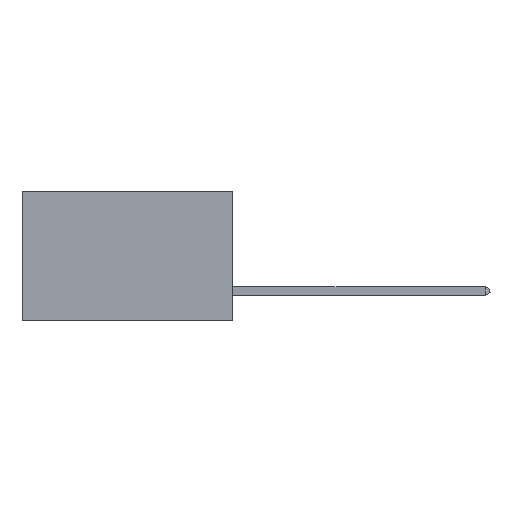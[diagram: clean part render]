
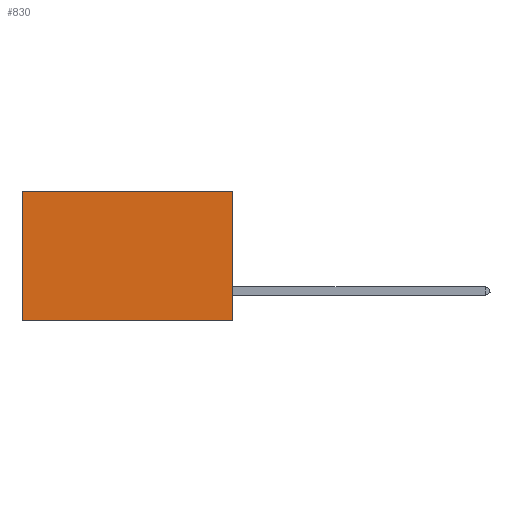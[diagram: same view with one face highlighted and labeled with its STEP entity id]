
A CAD part, left-side view. The second image highlights one B-rep face of the part: STEP entity #830.
In plain terms, the highlighted planar face has unit normal (-1, 0, 0).
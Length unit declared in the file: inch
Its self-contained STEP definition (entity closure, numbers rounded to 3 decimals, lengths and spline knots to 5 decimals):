
#830 = ADVANCED_FACE ( 'NONE', ( #8423 ), #7427, .F. ) ;
#2379 = VERTEX_POINT ( 'NONE', #4380 ) ;
#2841 = CARTESIAN_POINT ( 'NONE',  ( 0.2875, 0.6, 0. ) ) ;
#3124 = DIRECTION ( 'NONE',  ( 0., 1., 0. ) ) ;
#3214 = LINE ( 'NONE', #2841, #3964 ) ;
#3760 = EDGE_CURVE ( 'NONE', #12371, #2379, #3214, .T. ) ;
#3964 = VECTOR ( 'NONE', #4681, 39.37008 ) ;
#4380 = CARTESIAN_POINT ( 'NONE',  ( 0.2875, 0.6, -0.37 ) ) ;
#4681 = DIRECTION ( 'NONE',  ( 0., 0., -1. ) ) ;
#4777 = VERTEX_POINT ( 'NONE', #9364 ) ;
#4793 = EDGE_LOOP ( 'NONE', ( #9267, #10364, #8176, #6289 ) ) ;
#5035 = CARTESIAN_POINT ( 'NONE',  ( 0.2875, 0., -0.37 ) ) ;
#5230 = VECTOR ( 'NONE', #6561, 39.37008 ) ;
#5397 = CARTESIAN_POINT ( 'NONE',  ( 0.2875, 0., 0. ) ) ;
#5684 = VECTOR ( 'NONE', #11351, 39.37008 ) ;
#5814 = EDGE_CURVE ( 'NONE', #4777, #7488, #6009, .T. ) ;
#6009 = LINE ( 'NONE', #5397, #5684 ) ;
#6289 = ORIENTED_EDGE ( 'NONE', *, *, #12443, .T. ) ;
#6561 = DIRECTION ( 'NONE',  ( 0., 1., 0. ) ) ;
#6941 = AXIS2_PLACEMENT_3D ( 'NONE', #10407, #7470, #9533 ) ;
#7427 = PLANE ( 'NONE',  #6941 ) ;
#7435 = CARTESIAN_POINT ( 'NONE',  ( 0.2875, 0.6, 0. ) ) ;
#7470 = DIRECTION ( 'NONE',  ( 1., 0., 0. ) ) ;
#7488 = VERTEX_POINT ( 'NONE', #5035 ) ;
#8176 = ORIENTED_EDGE ( 'NONE', *, *, #5814, .F. ) ;
#8423 = FACE_OUTER_BOUND ( 'NONE', #4793, .T. ) ;
#8482 = CARTESIAN_POINT ( 'NONE',  ( 0.2875, 0., 0. ) ) ;
#9236 = EDGE_CURVE ( 'NONE', #7488, #2379, #10485, .T. ) ;
#9267 = ORIENTED_EDGE ( 'NONE', *, *, #3760, .T. ) ;
#9364 = CARTESIAN_POINT ( 'NONE',  ( 0.2875, 0., 0. ) ) ;
#9533 = DIRECTION ( 'NONE',  ( 0., 0., -1. ) ) ;
#10364 = ORIENTED_EDGE ( 'NONE', *, *, #9236, .F. ) ;
#10407 = CARTESIAN_POINT ( 'NONE',  ( 0.2875, 0., 0. ) ) ;
#10485 = LINE ( 'NONE', #10801, #11086 ) ;
#10801 = CARTESIAN_POINT ( 'NONE',  ( 0.2875, 0., -0.37 ) ) ;
#11086 = VECTOR ( 'NONE', #3124, 39.37008 ) ;
#11351 = DIRECTION ( 'NONE',  ( 0., 0., -1. ) ) ;
#11497 = LINE ( 'NONE', #8482, #5230 ) ;
#12371 = VERTEX_POINT ( 'NONE', #7435 ) ;
#12443 = EDGE_CURVE ( 'NONE', #4777, #12371, #11497, .T. ) ;
